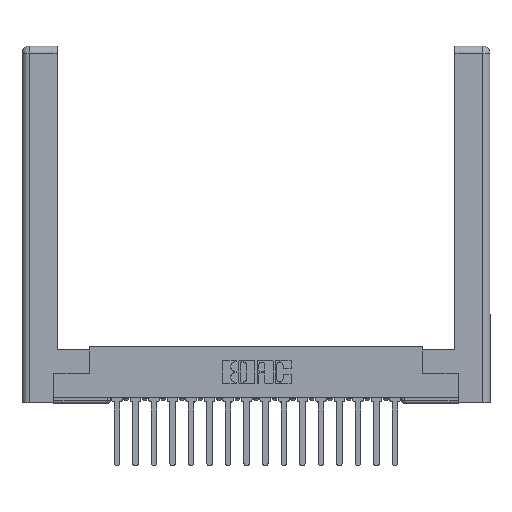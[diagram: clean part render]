
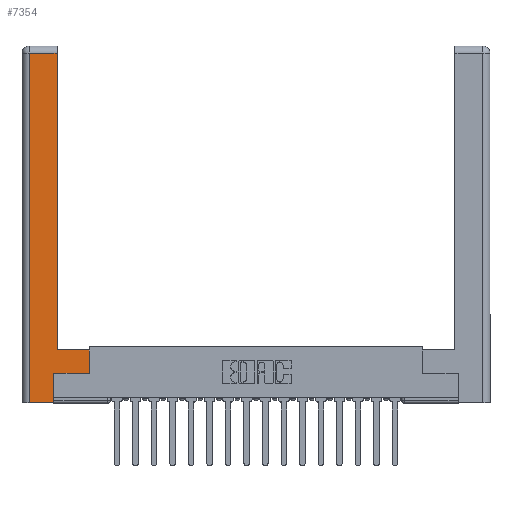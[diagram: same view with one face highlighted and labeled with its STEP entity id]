
A CAD part, top view. The second image highlights one B-rep face of the part: STEP entity #7354.
In plain terms, the highlighted planar face has unit normal (0, 0, 1).
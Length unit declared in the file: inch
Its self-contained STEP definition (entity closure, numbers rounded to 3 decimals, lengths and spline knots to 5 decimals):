
#232 = VERTEX_POINT ( 'NONE', #3581 ) ;
#548 = ORIENTED_EDGE ( 'NONE', *, *, #10623, .T. ) ;
#743 = LINE ( 'NONE', #18289, #6578 ) ;
#797 = CARTESIAN_POINT ( 'NONE',  ( 0.0615, 2.94, 0. ) ) ;
#1022 = DIRECTION ( 'NONE',  ( -1., 0., 0. ) ) ;
#1559 = LINE ( 'NONE', #4052, #2775 ) ;
#2752 = VECTOR ( 'NONE', #15999, 39.37008 ) ;
#2775 = VECTOR ( 'NONE', #8716, 39.37008 ) ;
#2915 = DIRECTION ( 'NONE',  ( 0., 0., -1. ) ) ;
#3016 = CARTESIAN_POINT ( 'NONE',  ( 0.565, 0.45, 0. ) ) ;
#3581 = CARTESIAN_POINT ( 'NONE',  ( 0.565, 0.45, 0. ) ) ;
#4052 = CARTESIAN_POINT ( 'NONE',  ( 0.265, 0.245, 0. ) ) ;
#4388 = ORIENTED_EDGE ( 'NONE', *, *, #15182, .T. ) ;
#4492 = LINE ( 'NONE', #16548, #10289 ) ;
#5023 = EDGE_LOOP ( 'NONE', ( #10742, #18554, #11035, #15592, #19474, #16017, #4388, #548 ) ) ;
#5046 = EDGE_CURVE ( 'NONE', #11739, #19579, #4492, .T. ) ;
#5111 = VERTEX_POINT ( 'NONE', #17963 ) ;
#5231 = LINE ( 'NONE', #11705, #8847 ) ;
#5361 = EDGE_CURVE ( 'NONE', #11454, #13232, #17748, .T. ) ;
#6578 = VECTOR ( 'NONE', #14972, 39.37008 ) ;
#7048 = VECTOR ( 'NONE', #16576, 39.37008 ) ;
#7354 = ADVANCED_FACE ( 'NONE', ( #19379 ), #16852, .F. ) ;
#7381 = DIRECTION ( 'NONE',  ( -1., 0., 0. ) ) ;
#7666 = CARTESIAN_POINT ( 'NONE',  ( 0.0615, 0., 0. ) ) ;
#7681 = VERTEX_POINT ( 'NONE', #14348 ) ;
#8124 = AXIS2_PLACEMENT_3D ( 'NONE', #16787, #2915, #10455 ) ;
#8244 = LINE ( 'NONE', #19610, #7048 ) ;
#8716 = DIRECTION ( 'NONE',  ( 0., 1., 0. ) ) ;
#8847 = VECTOR ( 'NONE', #18433, 39.37008 ) ;
#9897 = VERTEX_POINT ( 'NONE', #17967 ) ;
#9945 = EDGE_CURVE ( 'NONE', #13232, #5111, #1559, .T. ) ;
#10007 = EDGE_CURVE ( 'NONE', #7681, #11739, #5231, .T. ) ;
#10289 = VECTOR ( 'NONE', #7381, 39.37008 ) ;
#10455 = DIRECTION ( 'NONE',  ( -1., 0., 0. ) ) ;
#10623 = EDGE_CURVE ( 'NONE', #232, #7681, #18947, .T. ) ;
#10742 = ORIENTED_EDGE ( 'NONE', *, *, #10007, .T. ) ;
#11035 = ORIENTED_EDGE ( 'NONE', *, *, #17754, .T. ) ;
#11454 = VERTEX_POINT ( 'NONE', #7666 ) ;
#11500 = CARTESIAN_POINT ( 'NONE',  ( 0.265, 0., 0. ) ) ;
#11705 = CARTESIAN_POINT ( 'NONE',  ( 0.295, 3., 0. ) ) ;
#11739 = VERTEX_POINT ( 'NONE', #19096 ) ;
#11792 = LINE ( 'NONE', #3016, #14912 ) ;
#13232 = VERTEX_POINT ( 'NONE', #13373 ) ;
#13373 = CARTESIAN_POINT ( 'NONE',  ( 0.265, 0., 0. ) ) ;
#14348 = CARTESIAN_POINT ( 'NONE',  ( 0.295, 0.45, 0. ) ) ;
#14852 = VECTOR ( 'NONE', #1022, 39.37008 ) ;
#14912 = VECTOR ( 'NONE', #15460, 39.37008 ) ;
#14972 = DIRECTION ( 'NONE',  ( 0., -1., 0. ) ) ;
#15032 = CARTESIAN_POINT ( 'NONE',  ( 0.295, 0.45, 0. ) ) ;
#15182 = EDGE_CURVE ( 'NONE', #9897, #232, #11792, .T. ) ;
#15460 = DIRECTION ( 'NONE',  ( 0., 1., 0. ) ) ;
#15592 = ORIENTED_EDGE ( 'NONE', *, *, #5361, .T. ) ;
#15999 = DIRECTION ( 'NONE',  ( 1., 0., 0. ) ) ;
#16017 = ORIENTED_EDGE ( 'NONE', *, *, #18317, .T. ) ;
#16548 = CARTESIAN_POINT ( 'NONE',  ( 0.0615, 2.94, 0. ) ) ;
#16576 = DIRECTION ( 'NONE',  ( 1., 0., 0. ) ) ;
#16787 = CARTESIAN_POINT ( 'NONE',  ( 0., 0., 0. ) ) ;
#16852 = PLANE ( 'NONE',  #8124 ) ;
#17748 = LINE ( 'NONE', #11500, #2752 ) ;
#17754 = EDGE_CURVE ( 'NONE', #19579, #11454, #743, .T. ) ;
#17963 = CARTESIAN_POINT ( 'NONE',  ( 0.265, 0.245, 0. ) ) ;
#17967 = CARTESIAN_POINT ( 'NONE',  ( 0.565, 0.245, 0. ) ) ;
#18289 = CARTESIAN_POINT ( 'NONE',  ( 0.0615, 0., 0. ) ) ;
#18317 = EDGE_CURVE ( 'NONE', #5111, #9897, #8244, .T. ) ;
#18433 = DIRECTION ( 'NONE',  ( 0., 1., 0. ) ) ;
#18554 = ORIENTED_EDGE ( 'NONE', *, *, #5046, .T. ) ;
#18947 = LINE ( 'NONE', #15032, #14852 ) ;
#19096 = CARTESIAN_POINT ( 'NONE',  ( 0.295, 2.94, 0. ) ) ;
#19379 = FACE_OUTER_BOUND ( 'NONE', #5023, .T. ) ;
#19474 = ORIENTED_EDGE ( 'NONE', *, *, #9945, .T. ) ;
#19579 = VERTEX_POINT ( 'NONE', #797 ) ;
#19610 = CARTESIAN_POINT ( 'NONE',  ( 0.565, 0.245, 0. ) ) ;
